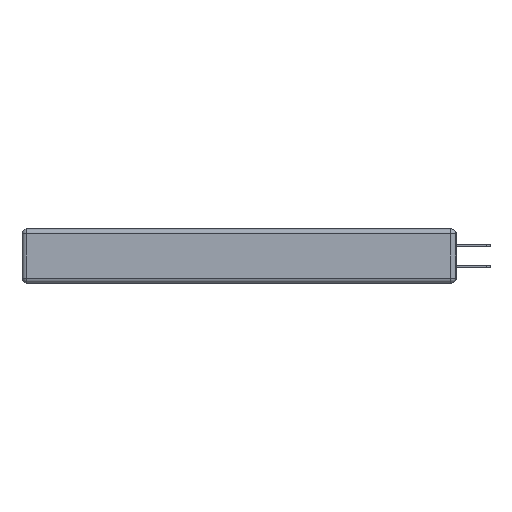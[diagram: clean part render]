
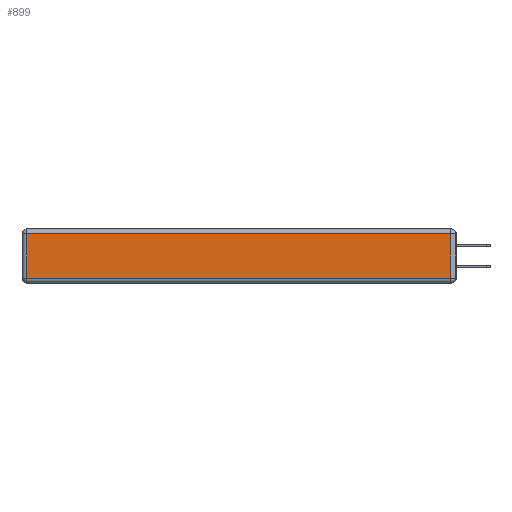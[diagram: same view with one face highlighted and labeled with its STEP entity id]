
A CAD part, left-side view. The second image highlights one B-rep face of the part: STEP entity #899.
In plain terms, the highlighted planar face has unit normal (-1, 0, 0).
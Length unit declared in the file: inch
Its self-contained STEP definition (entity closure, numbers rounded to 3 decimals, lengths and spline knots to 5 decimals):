
#5 = FACE_OUTER_BOUND ( 'NONE', #11722, .T. ) ;
#255 = EDGE_CURVE ( 'NONE', #2415, #17367, #877, .T. ) ;
#877 = LINE ( 'NONE', #10337, #2137 ) ;
#899 = ADVANCED_FACE ( 'NONE', ( #5 ), #14901, .T. ) ;
#1721 = ORIENTED_EDGE ( 'NONE', *, *, #2702, .T. ) ;
#2092 = VECTOR ( 'NONE', #14291, 39.37008 ) ;
#2137 = VECTOR ( 'NONE', #14468, 39.37008 ) ;
#2244 = VECTOR ( 'NONE', #10989, 39.37008 ) ;
#2307 = CARTESIAN_POINT ( 'NONE',  ( 0., 0.03, -0.343 ) ) ;
#2415 = VERTEX_POINT ( 'NONE', #15944 ) ;
#2702 = EDGE_CURVE ( 'NONE', #17367, #7340, #5372, .T. ) ;
#2831 = DIRECTION ( 'NONE',  ( 0., 1., 0. ) ) ;
#2889 = CARTESIAN_POINT ( 'NONE',  ( 0., 0., -0.343 ) ) ;
#3767 = CARTESIAN_POINT ( 'NONE',  ( 0., 0.03, -0.03 ) ) ;
#4985 = CARTESIAN_POINT ( 'NONE',  ( 0., 0., -0.313 ) ) ;
#5372 = LINE ( 'NONE', #4985, #2244 ) ;
#5651 = CARTESIAN_POINT ( 'NONE',  ( 0., 2.72, -0.313 ) ) ;
#5917 = CARTESIAN_POINT ( 'NONE',  ( 0., 0.03, -0.313 ) ) ;
#6259 = LINE ( 'NONE', #2307, #2092 ) ;
#7340 = VERTEX_POINT ( 'NONE', #5917 ) ;
#8245 = ORIENTED_EDGE ( 'NONE', *, *, #8746, .T. ) ;
#8746 = EDGE_CURVE ( 'NONE', #7340, #15885, #6259, .T. ) ;
#10081 = EDGE_CURVE ( 'NONE', #15885, #2415, #16757, .T. ) ;
#10337 = CARTESIAN_POINT ( 'NONE',  ( 0., 2.72, -0.343 ) ) ;
#10854 = CARTESIAN_POINT ( 'NONE',  ( 0., 2.75, -0.03 ) ) ;
#10989 = DIRECTION ( 'NONE',  ( 0., -1., 0. ) ) ;
#11051 = ORIENTED_EDGE ( 'NONE', *, *, #255, .T. ) ;
#11118 = DIRECTION ( 'NONE',  ( 0., 0., 1. ) ) ;
#11422 = AXIS2_PLACEMENT_3D ( 'NONE', #2889, #13641, #11118 ) ;
#11722 = EDGE_LOOP ( 'NONE', ( #1721, #8245, #13542, #11051 ) ) ;
#13542 = ORIENTED_EDGE ( 'NONE', *, *, #10081, .T. ) ;
#13641 = DIRECTION ( 'NONE',  ( -1., 0., 0. ) ) ;
#14225 = VECTOR ( 'NONE', #2831, 39.37008 ) ;
#14291 = DIRECTION ( 'NONE',  ( 0., 0., 1. ) ) ;
#14468 = DIRECTION ( 'NONE',  ( 0., 0., -1. ) ) ;
#14901 = PLANE ( 'NONE',  #11422 ) ;
#15885 = VERTEX_POINT ( 'NONE', #3767 ) ;
#15944 = CARTESIAN_POINT ( 'NONE',  ( 0., 2.72, -0.03 ) ) ;
#16757 = LINE ( 'NONE', #10854, #14225 ) ;
#17367 = VERTEX_POINT ( 'NONE', #5651 ) ;
